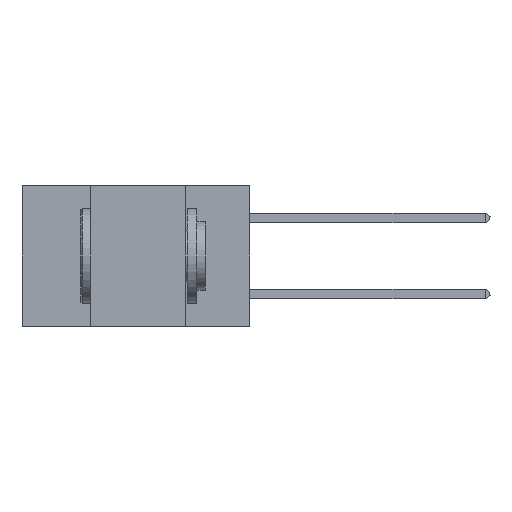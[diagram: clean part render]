
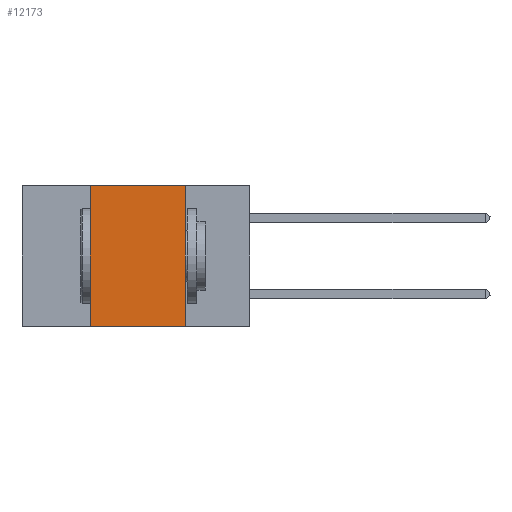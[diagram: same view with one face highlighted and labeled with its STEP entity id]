
A CAD part, left-side view. The second image highlights one B-rep face of the part: STEP entity #12173.
In plain terms, the highlighted planar face has unit normal (-1, 0, 0).
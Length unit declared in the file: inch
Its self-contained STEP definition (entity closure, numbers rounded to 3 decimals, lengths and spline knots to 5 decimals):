
#666 = VERTEX_POINT ( 'NONE', #43442 ) ;
#3147 = VECTOR ( 'NONE', #34121, 39.37008 ) ;
#3740 = AXIS2_PLACEMENT_3D ( 'NONE', #4442, #28615, #28760 ) ;
#4442 = CARTESIAN_POINT ( 'NONE',  ( 0., 0.6, 0. ) ) ;
#6012 = LINE ( 'NONE', #22613, #13027 ) ;
#6261 = EDGE_CURVE ( 'NONE', #36214, #9124, #6012, .T. ) ;
#6588 = LINE ( 'NONE', #19915, #22735 ) ;
#7805 = ORIENTED_EDGE ( 'NONE', *, *, #44701, .F. ) ;
#9124 = VERTEX_POINT ( 'NONE', #39325 ) ;
#12173 = ADVANCED_FACE ( 'NONE', ( #40567 ), #42252, .F. ) ;
#12513 = DIRECTION ( 'NONE',  ( 0., 0., -1. ) ) ;
#12976 = DIRECTION ( 'NONE',  ( 0., -1., 0. ) ) ;
#13027 = VECTOR ( 'NONE', #12513, 39.37008 ) ;
#16061 = CARTESIAN_POINT ( 'NONE',  ( 0., 0.17, 0. ) ) ;
#19636 = LINE ( 'NONE', #33569, #33731 ) ;
#19915 = CARTESIAN_POINT ( 'NONE',  ( 0., 0.6, 0. ) ) ;
#20426 = LINE ( 'NONE', #20594, #3147 ) ;
#20594 = CARTESIAN_POINT ( 'NONE',  ( 0., 0.42, 0. ) ) ;
#22613 = CARTESIAN_POINT ( 'NONE',  ( 0., 0.17, 0. ) ) ;
#22735 = VECTOR ( 'NONE', #12976, 39.37008 ) ;
#23224 = DIRECTION ( 'NONE',  ( 0., -1., 0. ) ) ;
#23779 = EDGE_CURVE ( 'NONE', #44784, #666, #20426, .T. ) ;
#25201 = ORIENTED_EDGE ( 'NONE', *, *, #27312, .T. ) ;
#27312 = EDGE_CURVE ( 'NONE', #44784, #9124, #19636, .T. ) ;
#28615 = DIRECTION ( 'NONE',  ( 1., 0., 0. ) ) ;
#28760 = DIRECTION ( 'NONE',  ( 0., 0., -1. ) ) ;
#33272 = ORIENTED_EDGE ( 'NONE', *, *, #6261, .F. ) ;
#33569 = CARTESIAN_POINT ( 'NONE',  ( 0., 0.6, -0.37 ) ) ;
#33731 = VECTOR ( 'NONE', #23224, 39.37008 ) ;
#34121 = DIRECTION ( 'NONE',  ( 0., 0., 1. ) ) ;
#36214 = VERTEX_POINT ( 'NONE', #16061 ) ;
#39014 = CARTESIAN_POINT ( 'NONE',  ( 0., 0.42, -0.37 ) ) ;
#39325 = CARTESIAN_POINT ( 'NONE',  ( 0., 0.17, -0.37 ) ) ;
#40567 = FACE_OUTER_BOUND ( 'NONE', #43576, .T. ) ;
#40958 = ORIENTED_EDGE ( 'NONE', *, *, #23779, .F. ) ;
#42252 = PLANE ( 'NONE',  #3740 ) ;
#43442 = CARTESIAN_POINT ( 'NONE',  ( 0., 0.42, 0. ) ) ;
#43576 = EDGE_LOOP ( 'NONE', ( #33272, #7805, #40958, #25201 ) ) ;
#44701 = EDGE_CURVE ( 'NONE', #666, #36214, #6588, .T. ) ;
#44784 = VERTEX_POINT ( 'NONE', #39014 ) ;
